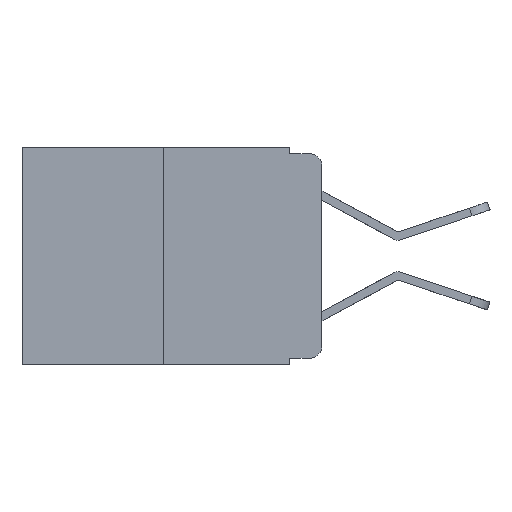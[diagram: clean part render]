
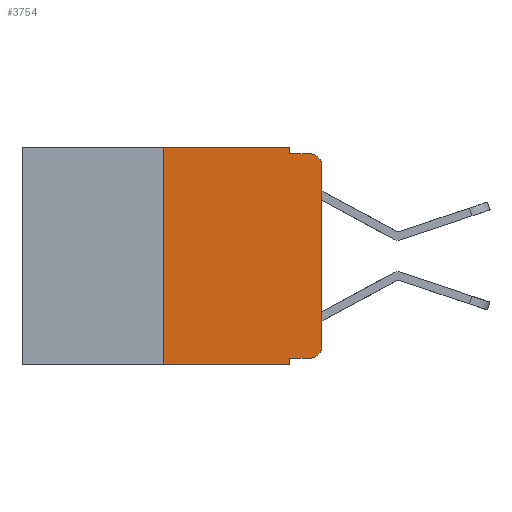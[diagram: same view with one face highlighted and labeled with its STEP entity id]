
A CAD part, left-side view. The second image highlights one B-rep face of the part: STEP entity #3754.
In plain terms, the highlighted planar face has unit normal (-1, 0, 0).
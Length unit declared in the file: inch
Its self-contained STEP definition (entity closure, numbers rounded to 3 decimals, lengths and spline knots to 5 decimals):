
#45 = CARTESIAN_POINT ( 'NONE',  ( 0., 0.473, 0. ) ) ;
#141 = CARTESIAN_POINT ( 'NONE',  ( 0., 0.25, -0.343 ) ) ;
#768 = DIRECTION ( 'NONE',  ( 0., 0., -1. ) ) ;
#965 = LINE ( 'NONE', #14465, #16684 ) ;
#1547 = EDGE_CURVE ( 'NONE', #15117, #18328, #8613, .T. ) ;
#1552 = DIRECTION ( 'NONE',  ( 0., 0., -1. ) ) ;
#1922 = DIRECTION ( 'NONE',  ( 0., -1., 0. ) ) ;
#2028 = VECTOR ( 'NONE', #18756, 39.37008 ) ;
#2264 = ORIENTED_EDGE ( 'NONE', *, *, #12251, .F. ) ;
#2295 = VECTOR ( 'NONE', #11285, 39.37008 ) ;
#2802 = LINE ( 'NONE', #14342, #2295 ) ;
#2979 = EDGE_CURVE ( 'NONE', #15411, #19389, #3866, .T. ) ;
#3170 = DIRECTION ( 'NONE',  ( 0., 0., -1. ) ) ;
#3228 = VECTOR ( 'NONE', #17382, 39.37008 ) ;
#3398 = EDGE_CURVE ( 'NONE', #14598, #19389, #965, .T. ) ;
#3559 = ORIENTED_EDGE ( 'NONE', *, *, #14691, .T. ) ;
#3563 = CARTESIAN_POINT ( 'NONE',  ( 0., 0.051, -0.343 ) ) ;
#3754 = ADVANCED_FACE ( 'NONE', ( #18081 ), #6091, .F. ) ;
#3866 = CIRCLE ( 'NONE', #5660, 0.02 ) ;
#3921 = VECTOR ( 'NONE', #9703, 39.37008 ) ;
#4235 = DIRECTION ( 'NONE',  ( 0., 0., 1. ) ) ;
#4242 = DIRECTION ( 'NONE',  ( -1., 0., 0. ) ) ;
#4375 = VERTEX_POINT ( 'NONE', #10947 ) ;
#4558 = ORIENTED_EDGE ( 'NONE', *, *, #19860, .T. ) ;
#4586 = CIRCLE ( 'NONE', #13532, 0.02 ) ;
#5176 = VECTOR ( 'NONE', #4235, 39.37008 ) ;
#5523 = ORIENTED_EDGE ( 'NONE', *, *, #2979, .T. ) ;
#5660 = AXIS2_PLACEMENT_3D ( 'NONE', #13530, #4242, #15074 ) ;
#5695 = CARTESIAN_POINT ( 'NONE',  ( 0., 0., 0. ) ) ;
#5748 = EDGE_CURVE ( 'NONE', #17125, #15117, #20149, .T. ) ;
#6091 = PLANE ( 'NONE',  #17282 ) ;
#6328 = LINE ( 'NONE', #8048, #2028 ) ;
#7480 = EDGE_CURVE ( 'NONE', #15194, #12976, #4586, .T. ) ;
#7620 = VECTOR ( 'NONE', #3170, 39.37008 ) ;
#7672 = DIRECTION ( 'NONE',  ( 0., 0., -1. ) ) ;
#7898 = CARTESIAN_POINT ( 'NONE',  ( 0., 0.051, 0. ) ) ;
#8048 = CARTESIAN_POINT ( 'NONE',  ( 0., 0.473, -0.343 ) ) ;
#8543 = LINE ( 'NONE', #9541, #16222 ) ;
#8613 = LINE ( 'NONE', #45, #3921 ) ;
#9333 = LINE ( 'NONE', #5695, #5176 ) ;
#9541 = CARTESIAN_POINT ( 'NONE',  ( 0., 0.051, 0. ) ) ;
#9703 = DIRECTION ( 'NONE',  ( 0., -1., 0. ) ) ;
#10347 = DIRECTION ( 'NONE',  ( -1., 0., 0. ) ) ;
#10947 = CARTESIAN_POINT ( 'NONE',  ( 0., 0.051, -0.333 ) ) ;
#11196 = EDGE_LOOP ( 'NONE', ( #16378, #5523, #18257, #13076, #13521, #15940, #4558, #2264, #3559, #13325 ) ) ;
#11253 = CARTESIAN_POINT ( 'NONE',  ( 0., 0., -0.313 ) ) ;
#11285 = DIRECTION ( 'NONE',  ( 0., -1., 0. ) ) ;
#12245 = CARTESIAN_POINT ( 'NONE',  ( 0., 0.473, 0. ) ) ;
#12251 = EDGE_CURVE ( 'NONE', #4375, #13032, #12691, .T. ) ;
#12691 = LINE ( 'NONE', #7898, #7620 ) ;
#12795 = CARTESIAN_POINT ( 'NONE',  ( 0., 0.25, 0. ) ) ;
#12976 = VERTEX_POINT ( 'NONE', #11253 ) ;
#13032 = VERTEX_POINT ( 'NONE', #3563 ) ;
#13076 = ORIENTED_EDGE ( 'NONE', *, *, #14601, .F. ) ;
#13325 = ORIENTED_EDGE ( 'NONE', *, *, #7480, .T. ) ;
#13521 = ORIENTED_EDGE ( 'NONE', *, *, #1547, .F. ) ;
#13530 = CARTESIAN_POINT ( 'NONE',  ( 0., 0.02, -0.03 ) ) ;
#13532 = AXIS2_PLACEMENT_3D ( 'NONE', #19489, #10347, #768 ) ;
#14342 = CARTESIAN_POINT ( 'NONE',  ( 0., 0.051, -0.333 ) ) ;
#14465 = CARTESIAN_POINT ( 'NONE',  ( 0., 0.051, -0.01 ) ) ;
#14598 = VERTEX_POINT ( 'NONE', #20199 ) ;
#14601 = EDGE_CURVE ( 'NONE', #18328, #14598, #8543, .T. ) ;
#14691 = EDGE_CURVE ( 'NONE', #4375, #15194, #2802, .T. ) ;
#14804 = CARTESIAN_POINT ( 'NONE',  ( 0., 0.051, 0. ) ) ;
#15074 = DIRECTION ( 'NONE',  ( 0., 0., -1. ) ) ;
#15117 = VERTEX_POINT ( 'NONE', #16858 ) ;
#15194 = VERTEX_POINT ( 'NONE', #20110 ) ;
#15411 = VERTEX_POINT ( 'NONE', #17460 ) ;
#15940 = ORIENTED_EDGE ( 'NONE', *, *, #5748, .F. ) ;
#16222 = VECTOR ( 'NONE', #1552, 39.37008 ) ;
#16378 = ORIENTED_EDGE ( 'NONE', *, *, #18452, .T. ) ;
#16684 = VECTOR ( 'NONE', #1922, 39.37008 ) ;
#16846 = DIRECTION ( 'NONE',  ( 1., 0., 0. ) ) ;
#16858 = CARTESIAN_POINT ( 'NONE',  ( 0., 0.25, 0. ) ) ;
#17125 = VERTEX_POINT ( 'NONE', #141 ) ;
#17282 = AXIS2_PLACEMENT_3D ( 'NONE', #12245, #16846, #7672 ) ;
#17382 = DIRECTION ( 'NONE',  ( 0., 0., 1. ) ) ;
#17460 = CARTESIAN_POINT ( 'NONE',  ( 0., 0., -0.03 ) ) ;
#17706 = CARTESIAN_POINT ( 'NONE',  ( 0., 0.02, -0.01 ) ) ;
#18081 = FACE_OUTER_BOUND ( 'NONE', #11196, .T. ) ;
#18257 = ORIENTED_EDGE ( 'NONE', *, *, #3398, .F. ) ;
#18328 = VERTEX_POINT ( 'NONE', #14804 ) ;
#18452 = EDGE_CURVE ( 'NONE', #12976, #15411, #9333, .T. ) ;
#18756 = DIRECTION ( 'NONE',  ( 0., -1., 0. ) ) ;
#19389 = VERTEX_POINT ( 'NONE', #17706 ) ;
#19489 = CARTESIAN_POINT ( 'NONE',  ( 0., 0.02, -0.313 ) ) ;
#19860 = EDGE_CURVE ( 'NONE', #17125, #13032, #6328, .T. ) ;
#20110 = CARTESIAN_POINT ( 'NONE',  ( 0., 0.02, -0.333 ) ) ;
#20149 = LINE ( 'NONE', #12795, #3228 ) ;
#20199 = CARTESIAN_POINT ( 'NONE',  ( 0., 0.051, -0.01 ) ) ;
